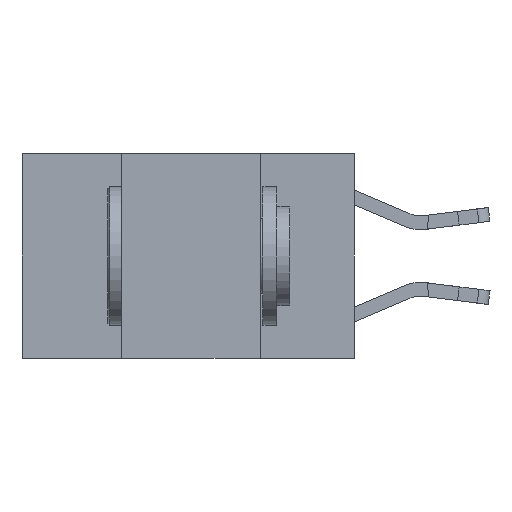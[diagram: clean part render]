
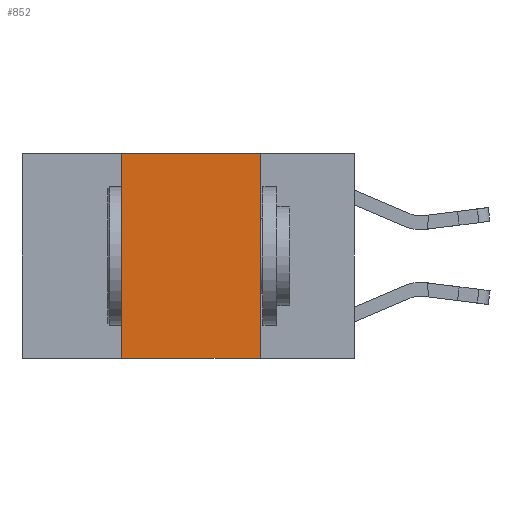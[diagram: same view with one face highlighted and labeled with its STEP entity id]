
A CAD part, left-side view. The second image highlights one B-rep face of the part: STEP entity #852.
In plain terms, the highlighted planar face has unit normal (-1, 0, 0).
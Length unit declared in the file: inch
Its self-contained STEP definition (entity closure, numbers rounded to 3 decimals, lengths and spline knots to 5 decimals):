
#185 = CARTESIAN_POINT ( 'NONE',  ( 0., 0.17, 0. ) ) ;
#852 = ADVANCED_FACE ( 'NONE', ( #6870 ), #9073, .F. ) ;
#1341 = CARTESIAN_POINT ( 'NONE',  ( 0., 0.42, 0. ) ) ;
#1414 = LINE ( 'NONE', #2378, #6554 ) ;
#2378 = CARTESIAN_POINT ( 'NONE',  ( 0., 0.42, 0. ) ) ;
#2397 = LINE ( 'NONE', #185, #12530 ) ;
#2818 = VERTEX_POINT ( 'NONE', #1341 ) ;
#3354 = VERTEX_POINT ( 'NONE', #3425 ) ;
#3368 = AXIS2_PLACEMENT_3D ( 'NONE', #5774, #10872, #7242 ) ;
#3425 = CARTESIAN_POINT ( 'NONE',  ( 0., 0.17, 0. ) ) ;
#4188 = ORIENTED_EDGE ( 'NONE', *, *, #9622, .F. ) ;
#4260 = DIRECTION ( 'NONE',  ( 0., -1., 0. ) ) ;
#4307 = EDGE_CURVE ( 'NONE', #12702, #7291, #7288, .T. ) ;
#4616 = EDGE_CURVE ( 'NONE', #12702, #2818, #1414, .T. ) ;
#5085 = CARTESIAN_POINT ( 'NONE',  ( 0., 0.17, -0.37 ) ) ;
#5774 = CARTESIAN_POINT ( 'NONE',  ( 0., 0.6, 0. ) ) ;
#6554 = VECTOR ( 'NONE', #11318, 39.37008 ) ;
#6870 = FACE_OUTER_BOUND ( 'NONE', #11358, .T. ) ;
#6932 = VECTOR ( 'NONE', #4260, 39.37008 ) ;
#7126 = CARTESIAN_POINT ( 'NONE',  ( 0., 0.42, -0.37 ) ) ;
#7222 = ORIENTED_EDGE ( 'NONE', *, *, #12353, .F. ) ;
#7242 = DIRECTION ( 'NONE',  ( 0., 0., -1. ) ) ;
#7288 = LINE ( 'NONE', #9385, #11936 ) ;
#7291 = VERTEX_POINT ( 'NONE', #5085 ) ;
#9073 = PLANE ( 'NONE',  #3368 ) ;
#9385 = CARTESIAN_POINT ( 'NONE',  ( 0., 0.6, -0.37 ) ) ;
#9622 = EDGE_CURVE ( 'NONE', #3354, #7291, #2397, .T. ) ;
#9836 = DIRECTION ( 'NONE',  ( 0., 0., -1. ) ) ;
#9855 = LINE ( 'NONE', #10851, #6932 ) ;
#10851 = CARTESIAN_POINT ( 'NONE',  ( 0., 0.6, 0. ) ) ;
#10872 = DIRECTION ( 'NONE',  ( 1., 0., 0. ) ) ;
#11318 = DIRECTION ( 'NONE',  ( 0., 0., 1. ) ) ;
#11320 = ORIENTED_EDGE ( 'NONE', *, *, #4307, .T. ) ;
#11358 = EDGE_LOOP ( 'NONE', ( #4188, #7222, #12712, #11320 ) ) ;
#11936 = VECTOR ( 'NONE', #12634, 39.37008 ) ;
#12353 = EDGE_CURVE ( 'NONE', #2818, #3354, #9855, .T. ) ;
#12530 = VECTOR ( 'NONE', #9836, 39.37008 ) ;
#12634 = DIRECTION ( 'NONE',  ( 0., -1., 0. ) ) ;
#12702 = VERTEX_POINT ( 'NONE', #7126 ) ;
#12712 = ORIENTED_EDGE ( 'NONE', *, *, #4616, .F. ) ;
